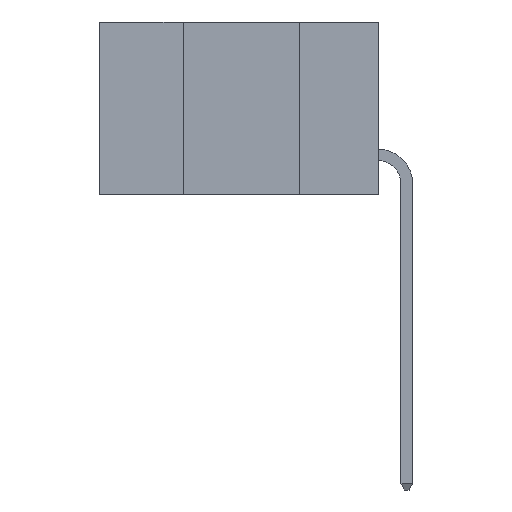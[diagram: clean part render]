
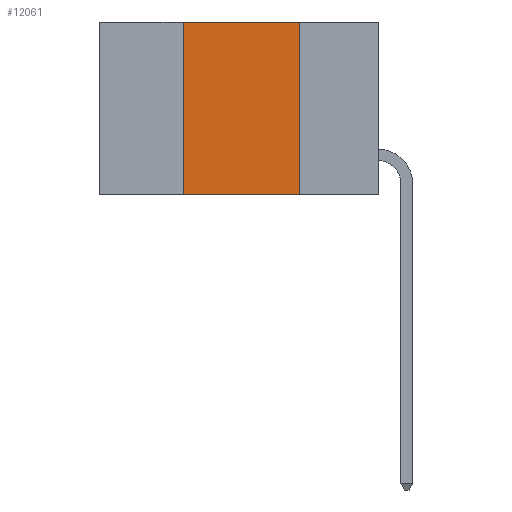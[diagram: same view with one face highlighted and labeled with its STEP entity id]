
A CAD part, left-side view. The second image highlights one B-rep face of the part: STEP entity #12061.
In plain terms, the highlighted planar face has unit normal (-1, 0, 0).
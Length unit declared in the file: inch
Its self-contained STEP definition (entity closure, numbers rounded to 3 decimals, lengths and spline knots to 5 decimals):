
#300 = CARTESIAN_POINT ( 'NONE',  ( 0., 0.6, 0. ) ) ;
#1053 = EDGE_CURVE ( 'NONE', #18819, #19289, #3963, .T. ) ;
#1065 = VERTEX_POINT ( 'NONE', #13344 ) ;
#1602 = VERTEX_POINT ( 'NONE', #16895 ) ;
#1658 = PLANE ( 'NONE',  #15838 ) ;
#2622 = ORIENTED_EDGE ( 'NONE', *, *, #8402, .T. ) ;
#3282 = DIRECTION ( 'NONE',  ( 1., 0., 0. ) ) ;
#3653 = LINE ( 'NONE', #12835, #20018 ) ;
#3963 = LINE ( 'NONE', #15813, #13085 ) ;
#4046 = EDGE_LOOP ( 'NONE', ( #12441, #10436, #14913, #2622 ) ) ;
#4166 = CARTESIAN_POINT ( 'NONE',  ( 0., 0.17, -0.37 ) ) ;
#7500 = EDGE_CURVE ( 'NONE', #1602, #1065, #13306, .T. ) ;
#8164 = CARTESIAN_POINT ( 'NONE',  ( 0., 0.6, 0. ) ) ;
#8402 = EDGE_CURVE ( 'NONE', #18819, #1065, #3653, .T. ) ;
#10094 = CARTESIAN_POINT ( 'NONE',  ( 0., 0.42, -0.37 ) ) ;
#10436 = ORIENTED_EDGE ( 'NONE', *, *, #12173, .F. ) ;
#10915 = DIRECTION ( 'NONE',  ( 0., 0., 1. ) ) ;
#11240 = DIRECTION ( 'NONE',  ( 0., -1., 0. ) ) ;
#12061 = ADVANCED_FACE ( 'NONE', ( #14789 ), #1658, .F. ) ;
#12173 = EDGE_CURVE ( 'NONE', #19289, #1602, #16494, .T. ) ;
#12441 = ORIENTED_EDGE ( 'NONE', *, *, #7500, .F. ) ;
#12835 = CARTESIAN_POINT ( 'NONE',  ( 0., 0.6, -0.37 ) ) ;
#13085 = VECTOR ( 'NONE', #10915, 39.37008 ) ;
#13248 = DIRECTION ( 'NONE',  ( 0., -1., 0. ) ) ;
#13306 = LINE ( 'NONE', #4166, #17505 ) ;
#13344 = CARTESIAN_POINT ( 'NONE',  ( 0., 0.17, -0.37 ) ) ;
#14391 = CARTESIAN_POINT ( 'NONE',  ( 0., 0.42, 0. ) ) ;
#14582 = DIRECTION ( 'NONE',  ( 0., 0., -1. ) ) ;
#14789 = FACE_OUTER_BOUND ( 'NONE', #4046, .T. ) ;
#14913 = ORIENTED_EDGE ( 'NONE', *, *, #1053, .F. ) ;
#15813 = CARTESIAN_POINT ( 'NONE',  ( 0., 0.42, -0.37 ) ) ;
#15838 = AXIS2_PLACEMENT_3D ( 'NONE', #8164, #3282, #14582 ) ;
#16494 = LINE ( 'NONE', #300, #16971 ) ;
#16895 = CARTESIAN_POINT ( 'NONE',  ( 0., 0.17, 0. ) ) ;
#16971 = VECTOR ( 'NONE', #13248, 39.37008 ) ;
#17505 = VECTOR ( 'NONE', #19969, 39.37008 ) ;
#18819 = VERTEX_POINT ( 'NONE', #10094 ) ;
#19289 = VERTEX_POINT ( 'NONE', #14391 ) ;
#19969 = DIRECTION ( 'NONE',  ( 0., 0., -1. ) ) ;
#20018 = VECTOR ( 'NONE', #11240, 39.37008 ) ;
